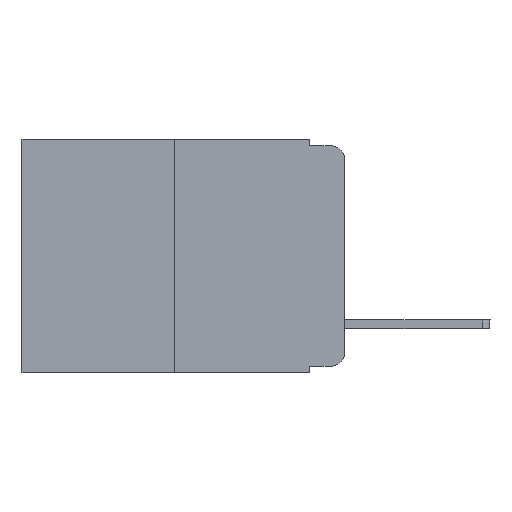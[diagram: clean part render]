
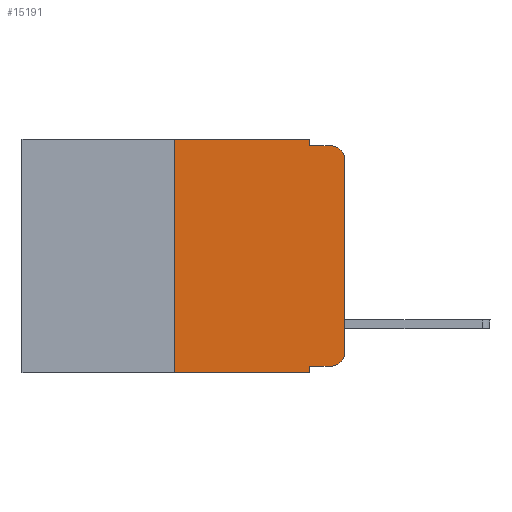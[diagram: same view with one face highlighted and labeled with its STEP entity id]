
A CAD part, left-side view. The second image highlights one B-rep face of the part: STEP entity #15191.
In plain terms, the highlighted planar face has unit normal (-1, 0, 0).
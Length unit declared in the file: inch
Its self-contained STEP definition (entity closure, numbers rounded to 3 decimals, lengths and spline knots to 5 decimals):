
#408 = CARTESIAN_POINT ( 'NONE',  ( 0., 0., 0. ) ) ;
#731 = ORIENTED_EDGE ( 'NONE', *, *, #12874, .F. ) ;
#752 = AXIS2_PLACEMENT_3D ( 'NONE', #17750, #21168, #9418 ) ;
#1680 = CARTESIAN_POINT ( 'NONE',  ( 0., 0., -0.03 ) ) ;
#1730 = CARTESIAN_POINT ( 'NONE',  ( 0., 0.051, 0. ) ) ;
#2065 = EDGE_CURVE ( 'NONE', #16933, #3653, #13995, .T. ) ;
#2454 = EDGE_CURVE ( 'NONE', #20531, #20631, #11810, .T. ) ;
#2649 = DIRECTION ( 'NONE',  ( 0., -1., 0. ) ) ;
#3463 = VERTEX_POINT ( 'NONE', #7278 ) ;
#3475 = LINE ( 'NONE', #11495, #7251 ) ;
#3500 = DIRECTION ( 'NONE',  ( 0., 0., -1. ) ) ;
#3603 = CARTESIAN_POINT ( 'NONE',  ( 0., 0.473, -0.343 ) ) ;
#3653 = VERTEX_POINT ( 'NONE', #4294 ) ;
#3967 = DIRECTION ( 'NONE',  ( 0., 0., 1. ) ) ;
#4294 = CARTESIAN_POINT ( 'NONE',  ( 0., 0., -0.313 ) ) ;
#4523 = VERTEX_POINT ( 'NONE', #1680 ) ;
#4799 = ORIENTED_EDGE ( 'NONE', *, *, #21177, .F. ) ;
#5186 = DIRECTION ( 'NONE',  ( 0., 0., -1. ) ) ;
#5238 = DIRECTION ( 'NONE',  ( 0., 0., -1. ) ) ;
#5375 = CARTESIAN_POINT ( 'NONE',  ( 0., 0.25, 0. ) ) ;
#6382 = ORIENTED_EDGE ( 'NONE', *, *, #20378, .F. ) ;
#6990 = VECTOR ( 'NONE', #15462, 39.37008 ) ;
#7014 = ORIENTED_EDGE ( 'NONE', *, *, #2454, .F. ) ;
#7111 = DIRECTION ( 'NONE',  ( 0., 0., 1. ) ) ;
#7144 = DIRECTION ( 'NONE',  ( -1., 0., 0. ) ) ;
#7251 = VECTOR ( 'NONE', #20056, 39.37008 ) ;
#7278 = CARTESIAN_POINT ( 'NONE',  ( 0., 0.051, 0. ) ) ;
#7914 = VECTOR ( 'NONE', #3967, 39.37008 ) ;
#7967 = ORIENTED_EDGE ( 'NONE', *, *, #2065, .T. ) ;
#8367 = ORIENTED_EDGE ( 'NONE', *, *, #9609, .T. ) ;
#9418 = DIRECTION ( 'NONE',  ( 0., 0., -1. ) ) ;
#9531 = VECTOR ( 'NONE', #19603, 39.37008 ) ;
#9609 = EDGE_CURVE ( 'NONE', #3653, #4523, #15443, .T. ) ;
#10050 = VERTEX_POINT ( 'NONE', #13410 ) ;
#10108 = ORIENTED_EDGE ( 'NONE', *, *, #10736, .T. ) ;
#10736 = EDGE_CURVE ( 'NONE', #21042, #20631, #18641, .T. ) ;
#10904 = CARTESIAN_POINT ( 'NONE',  ( 0., 0.02, -0.333 ) ) ;
#10943 = CARTESIAN_POINT ( 'NONE',  ( 0., 0.25, -0.343 ) ) ;
#11451 = EDGE_CURVE ( 'NONE', #4523, #19296, #12395, .T. ) ;
#11495 = CARTESIAN_POINT ( 'NONE',  ( 0., 0.051, 0. ) ) ;
#11759 = DIRECTION ( 'NONE',  ( -1., 0., 0. ) ) ;
#11810 = LINE ( 'NONE', #1730, #16099 ) ;
#11879 = VECTOR ( 'NONE', #2649, 39.37008 ) ;
#12034 = ORIENTED_EDGE ( 'NONE', *, *, #11451, .T. ) ;
#12340 = ORIENTED_EDGE ( 'NONE', *, *, #15354, .F. ) ;
#12395 = CIRCLE ( 'NONE', #18019, 0.02 ) ;
#12515 = CARTESIAN_POINT ( 'NONE',  ( 0., 0.051, -0.01 ) ) ;
#12874 = EDGE_CURVE ( 'NONE', #10050, #19296, #20871, .T. ) ;
#13050 = EDGE_CURVE ( 'NONE', #20531, #16933, #18546, .T. ) ;
#13206 = VERTEX_POINT ( 'NONE', #5375 ) ;
#13410 = CARTESIAN_POINT ( 'NONE',  ( 0., 0.051, -0.01 ) ) ;
#13636 = LINE ( 'NONE', #20323, #7914 ) ;
#13995 = CIRCLE ( 'NONE', #18555, 0.02 ) ;
#14026 = PLANE ( 'NONE',  #752 ) ;
#15191 = ADVANCED_FACE ( 'NONE', ( #15985 ), #14026, .F. ) ;
#15262 = CARTESIAN_POINT ( 'NONE',  ( 0., 0.02, -0.313 ) ) ;
#15354 = EDGE_CURVE ( 'NONE', #13206, #3463, #21602, .T. ) ;
#15443 = LINE ( 'NONE', #408, #21655 ) ;
#15462 = DIRECTION ( 'NONE',  ( 0., -1., 0. ) ) ;
#15985 = FACE_OUTER_BOUND ( 'NONE', #17663, .T. ) ;
#16099 = VECTOR ( 'NONE', #5238, 39.37008 ) ;
#16200 = ORIENTED_EDGE ( 'NONE', *, *, #13050, .T. ) ;
#16248 = CARTESIAN_POINT ( 'NONE',  ( 0., 0.02, -0.01 ) ) ;
#16466 = CARTESIAN_POINT ( 'NONE',  ( 0., 0.051, -0.333 ) ) ;
#16651 = CARTESIAN_POINT ( 'NONE',  ( 0., 0.473, 0. ) ) ;
#16933 = VERTEX_POINT ( 'NONE', #10904 ) ;
#17663 = EDGE_LOOP ( 'NONE', ( #8367, #12034, #731, #4799, #12340, #6382, #10108, #7014, #16200, #7967 ) ) ;
#17750 = CARTESIAN_POINT ( 'NONE',  ( 0., 0.473, 0. ) ) ;
#17898 = CARTESIAN_POINT ( 'NONE',  ( 0., 0.051, -0.343 ) ) ;
#18019 = AXIS2_PLACEMENT_3D ( 'NONE', #19996, #11759, #5186 ) ;
#18546 = LINE ( 'NONE', #16466, #19957 ) ;
#18555 = AXIS2_PLACEMENT_3D ( 'NONE', #15262, #7144, #3500 ) ;
#18641 = LINE ( 'NONE', #3603, #6990 ) ;
#19296 = VERTEX_POINT ( 'NONE', #16248 ) ;
#19427 = CARTESIAN_POINT ( 'NONE',  ( 0., 0.051, -0.333 ) ) ;
#19603 = DIRECTION ( 'NONE',  ( 0., -1., 0. ) ) ;
#19957 = VECTOR ( 'NONE', #20088, 39.37008 ) ;
#19996 = CARTESIAN_POINT ( 'NONE',  ( 0., 0.02, -0.03 ) ) ;
#20056 = DIRECTION ( 'NONE',  ( 0., 0., -1. ) ) ;
#20088 = DIRECTION ( 'NONE',  ( 0., -1., 0. ) ) ;
#20323 = CARTESIAN_POINT ( 'NONE',  ( 0., 0.25, 0. ) ) ;
#20378 = EDGE_CURVE ( 'NONE', #21042, #13206, #13636, .T. ) ;
#20531 = VERTEX_POINT ( 'NONE', #19427 ) ;
#20631 = VERTEX_POINT ( 'NONE', #17898 ) ;
#20871 = LINE ( 'NONE', #12515, #11879 ) ;
#21042 = VERTEX_POINT ( 'NONE', #10943 ) ;
#21168 = DIRECTION ( 'NONE',  ( 1., 0., 0. ) ) ;
#21177 = EDGE_CURVE ( 'NONE', #3463, #10050, #3475, .T. ) ;
#21602 = LINE ( 'NONE', #16651, #9531 ) ;
#21655 = VECTOR ( 'NONE', #7111, 39.37008 ) ;
